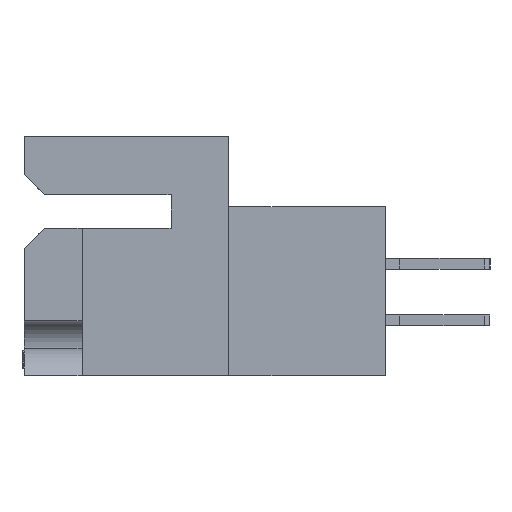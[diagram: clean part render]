
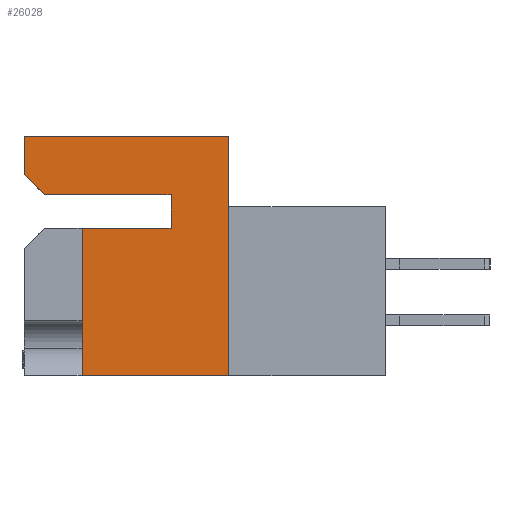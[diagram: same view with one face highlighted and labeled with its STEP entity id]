
A CAD part, left-side view. The second image highlights one B-rep face of the part: STEP entity #26028.
In plain terms, the highlighted planar face has unit normal (-1, 0, 0).
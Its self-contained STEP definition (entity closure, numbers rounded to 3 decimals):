
#154 = ORIENTED_EDGE ( 'NONE', *, *, #15219, .F. ) ;
#200 = EDGE_CURVE ( 'NONE', #34109, #506, #8387, .T. ) ;
#404 = CARTESIAN_POINT ( 'NONE',  ( 0., 8.255, -13.487 ) ) ;
#442 = LINE ( 'NONE', #17573, #1293 ) ;
#506 = VERTEX_POINT ( 'NONE', #32653 ) ;
#874 = CARTESIAN_POINT ( 'NONE',  ( 0., 10.363, -3.302 ) ) ;
#1293 = VECTOR ( 'NONE', #12321, 1000. ) ;
#3405 = ORIENTED_EDGE ( 'NONE', *, *, #25251, .F. ) ;
#3454 = DIRECTION ( 'NONE',  ( 1., 0., 0. ) ) ;
#4378 = ORIENTED_EDGE ( 'NONE', *, *, #17293, .F. ) ;
#4736 = DIRECTION ( 'NONE',  ( 0., 1., 0. ) ) ;
#5149 = DIRECTION ( 'NONE',  ( 0., -1., 0. ) ) ;
#5197 = VECTOR ( 'NONE', #30162, 1000. ) ;
#5239 = ORIENTED_EDGE ( 'NONE', *, *, #200, .F. ) ;
#5282 = LINE ( 'NONE', #21003, #18870 ) ;
#5472 = CARTESIAN_POINT ( 'NONE',  ( 0., 0., 0. ) ) ;
#5488 = AXIS2_PLACEMENT_3D ( 'NONE', #5472, #3454, #15630 ) ;
#6924 = EDGE_LOOP ( 'NONE', ( #19231, #9702, #154, #5239, #25094, #3405, #7150, #16452, #4378 ) ) ;
#6946 = VECTOR ( 'NONE', #34176, 1000. ) ;
#6975 = EDGE_CURVE ( 'NONE', #34109, #27365, #442, .T. ) ;
#7150 = ORIENTED_EDGE ( 'NONE', *, *, #17508, .F. ) ;
#7731 = CARTESIAN_POINT ( 'NONE',  ( 0., 11.506, 0. ) ) ;
#7753 = LINE ( 'NONE', #16528, #20504 ) ;
#8387 = LINE ( 'NONE', #19891, #21616 ) ;
#9702 = ORIENTED_EDGE ( 'NONE', *, *, #10123, .F. ) ;
#10093 = FACE_OUTER_BOUND ( 'NONE', #6924, .T. ) ;
#10123 = EDGE_CURVE ( 'NONE', #22241, #29281, #33863, .T. ) ;
#10659 = PLANE ( 'NONE',  #5488 ) ;
#10681 = LINE ( 'NONE', #27413, #5197 ) ;
#11017 = LINE ( 'NONE', #11376, #16947 ) ;
#11376 = CARTESIAN_POINT ( 'NONE',  ( 0., 0., -3.302 ) ) ;
#12321 = DIRECTION ( 'NONE',  ( 0., -0.707, -0.707 ) ) ;
#12521 = EDGE_CURVE ( 'NONE', #13439, #32766, #10681, .T. ) ;
#13439 = VERTEX_POINT ( 'NONE', #28887 ) ;
#14153 = LINE ( 'NONE', #18313, #6946 ) ;
#15219 = EDGE_CURVE ( 'NONE', #506, #22241, #32768, .T. ) ;
#15630 = DIRECTION ( 'NONE',  ( 0., 0., -1. ) ) ;
#16452 = ORIENTED_EDGE ( 'NONE', *, *, #12521, .F. ) ;
#16528 = CARTESIAN_POINT ( 'NONE',  ( 0., 3.251, -5.182 ) ) ;
#16947 = VECTOR ( 'NONE', #19472, 1000. ) ;
#17293 = EDGE_CURVE ( 'NONE', #25280, #13439, #14153, .T. ) ;
#17508 = EDGE_CURVE ( 'NONE', #32766, #32956, #7753, .T. ) ;
#17573 = CARTESIAN_POINT ( 'NONE',  ( 0., 10.363, -3.302 ) ) ;
#17594 = DIRECTION ( 'NONE',  ( 0., 0., -1. ) ) ;
#18048 = CARTESIAN_POINT ( 'NONE',  ( 0., 11.506, -2.159 ) ) ;
#18313 = CARTESIAN_POINT ( 'NONE',  ( 0., 8.255, -5.182 ) ) ;
#18659 = CARTESIAN_POINT ( 'NONE',  ( 0., 0., -13.487 ) ) ;
#18870 = VECTOR ( 'NONE', #4736, 1000. ) ;
#19231 = ORIENTED_EDGE ( 'NONE', *, *, #34700, .F. ) ;
#19472 = DIRECTION ( 'NONE',  ( 0., 1., 0. ) ) ;
#19891 = CARTESIAN_POINT ( 'NONE',  ( 0., 11.506, -13.487 ) ) ;
#20504 = VECTOR ( 'NONE', #24509, 1000. ) ;
#21003 = CARTESIAN_POINT ( 'NONE',  ( 0., -8.814, -13.487 ) ) ;
#21616 = VECTOR ( 'NONE', #22651, 1000. ) ;
#22241 = VERTEX_POINT ( 'NONE', #26955 ) ;
#22651 = DIRECTION ( 'NONE',  ( 0., 0., 1. ) ) ;
#22796 = VECTOR ( 'NONE', #17594, 1000. ) ;
#24509 = DIRECTION ( 'NONE',  ( 0., 0., 1. ) ) ;
#24657 = CARTESIAN_POINT ( 'NONE',  ( 0., 3.251, -5.182 ) ) ;
#25094 = ORIENTED_EDGE ( 'NONE', *, *, #6975, .T. ) ;
#25251 = EDGE_CURVE ( 'NONE', #32956, #27365, #11017, .T. ) ;
#25280 = VERTEX_POINT ( 'NONE', #404 ) ;
#25492 = VECTOR ( 'NONE', #5149, 1000. ) ;
#26028 = ADVANCED_FACE ( 'NONE', ( #10093 ), #10659, .F. ) ;
#26955 = CARTESIAN_POINT ( 'NONE',  ( 0., 0., 0. ) ) ;
#27365 = VERTEX_POINT ( 'NONE', #874 ) ;
#27413 = CARTESIAN_POINT ( 'NONE',  ( 0., 0., -5.182 ) ) ;
#28482 = CARTESIAN_POINT ( 'NONE',  ( 0., 0., 0. ) ) ;
#28887 = CARTESIAN_POINT ( 'NONE',  ( 0., 8.255, -5.182 ) ) ;
#29281 = VERTEX_POINT ( 'NONE', #18659 ) ;
#30162 = DIRECTION ( 'NONE',  ( 0., -1., 0. ) ) ;
#30169 = CARTESIAN_POINT ( 'NONE',  ( 0., 3.251, -3.302 ) ) ;
#32653 = CARTESIAN_POINT ( 'NONE',  ( 0., 11.506, 0. ) ) ;
#32766 = VERTEX_POINT ( 'NONE', #24657 ) ;
#32768 = LINE ( 'NONE', #7731, #25492 ) ;
#32956 = VERTEX_POINT ( 'NONE', #30169 ) ;
#33863 = LINE ( 'NONE', #28482, #22796 ) ;
#34109 = VERTEX_POINT ( 'NONE', #18048 ) ;
#34176 = DIRECTION ( 'NONE',  ( 0., 0., 1. ) ) ;
#34700 = EDGE_CURVE ( 'NONE', #29281, #25280, #5282, .T. ) ;
